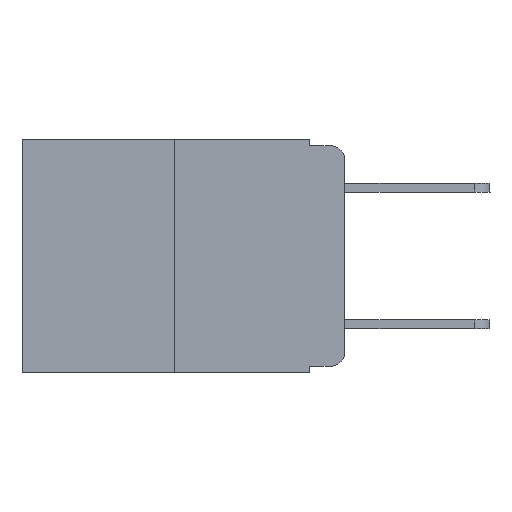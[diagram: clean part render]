
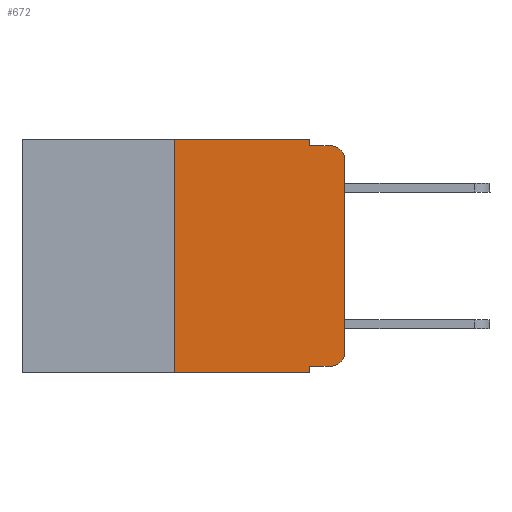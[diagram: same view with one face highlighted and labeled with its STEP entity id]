
A CAD part, left-side view. The second image highlights one B-rep face of the part: STEP entity #672.
In plain terms, the highlighted planar face has unit normal (-1, 0, 0).
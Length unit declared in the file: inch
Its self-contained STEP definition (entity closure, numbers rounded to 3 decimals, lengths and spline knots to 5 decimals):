
#62 = DIRECTION ( 'NONE',  ( 0., 0., -1. ) ) ;
#180 = DIRECTION ( 'NONE',  ( 0., -1., 0. ) ) ;
#603 = CARTESIAN_POINT ( 'NONE',  ( 0., 0.25, 0. ) ) ;
#672 = ADVANCED_FACE ( 'NONE', ( #15257 ), #4066, .F. ) ;
#681 = ORIENTED_EDGE ( 'NONE', *, *, #3427, .F. ) ;
#793 = DIRECTION ( 'NONE',  ( 0., 0., -1. ) ) ;
#1193 = DIRECTION ( 'NONE',  ( -1., 0., 0. ) ) ;
#1286 = VECTOR ( 'NONE', #15702, 39.37008 ) ;
#1287 = CARTESIAN_POINT ( 'NONE',  ( 0., 0., 0. ) ) ;
#1484 = LINE ( 'NONE', #16056, #1286 ) ;
#1562 = CARTESIAN_POINT ( 'NONE',  ( 0., 0.25, -0.343 ) ) ;
#1716 = VERTEX_POINT ( 'NONE', #8969 ) ;
#1784 = VECTOR ( 'NONE', #18478, 39.37008 ) ;
#2101 = ORIENTED_EDGE ( 'NONE', *, *, #10340, .T. ) ;
#2102 = LINE ( 'NONE', #6724, #8896 ) ;
#3020 = CARTESIAN_POINT ( 'NONE',  ( 0., 0.051, 0. ) ) ;
#3427 = EDGE_CURVE ( 'NONE', #9425, #6986, #13265, .T. ) ;
#3768 = CIRCLE ( 'NONE', #14572, 0.02 ) ;
#4066 = PLANE ( 'NONE',  #12534 ) ;
#4301 = DIRECTION ( 'NONE',  ( 0., 0., -1. ) ) ;
#4521 = DIRECTION ( 'NONE',  ( 0., 0., -1. ) ) ;
#4701 = ORIENTED_EDGE ( 'NONE', *, *, #14159, .F. ) ;
#5406 = EDGE_CURVE ( 'NONE', #7243, #9425, #1484, .T. ) ;
#5441 = AXIS2_PLACEMENT_3D ( 'NONE', #14622, #12945, #4301 ) ;
#5996 = VERTEX_POINT ( 'NONE', #9177 ) ;
#6724 = CARTESIAN_POINT ( 'NONE',  ( 0., 0.051, 0. ) ) ;
#6986 = VERTEX_POINT ( 'NONE', #16892 ) ;
#7062 = EDGE_CURVE ( 'NONE', #7435, #14889, #14156, .T. ) ;
#7243 = VERTEX_POINT ( 'NONE', #603 ) ;
#7412 = CARTESIAN_POINT ( 'NONE',  ( 0., 0.02, -0.01 ) ) ;
#7435 = VERTEX_POINT ( 'NONE', #9754 ) ;
#7472 = LINE ( 'NONE', #14248, #10600 ) ;
#7622 = LINE ( 'NONE', #11838, #1784 ) ;
#7939 = CARTESIAN_POINT ( 'NONE',  ( 0., 0., -0.03 ) ) ;
#8107 = EDGE_CURVE ( 'NONE', #14889, #14219, #15342, .T. ) ;
#8110 = DIRECTION ( 'NONE',  ( 1., 0., 0. ) ) ;
#8122 = VERTEX_POINT ( 'NONE', #1562 ) ;
#8605 = VECTOR ( 'NONE', #15674, 39.37008 ) ;
#8896 = VECTOR ( 'NONE', #793, 39.37008 ) ;
#8969 = CARTESIAN_POINT ( 'NONE',  ( 0., 0.051, -0.333 ) ) ;
#9177 = CARTESIAN_POINT ( 'NONE',  ( 0., 0.051, -0.343 ) ) ;
#9425 = VERTEX_POINT ( 'NONE', #13132 ) ;
#9754 = CARTESIAN_POINT ( 'NONE',  ( 0., 0., -0.313 ) ) ;
#9909 = EDGE_CURVE ( 'NONE', #8122, #7243, #7472, .T. ) ;
#10340 = EDGE_CURVE ( 'NONE', #8122, #5996, #7622, .T. ) ;
#10359 = ORIENTED_EDGE ( 'NONE', *, *, #14154, .T. ) ;
#10519 = CARTESIAN_POINT ( 'NONE',  ( 0., 0.051, -0.333 ) ) ;
#10600 = VECTOR ( 'NONE', #17154, 39.37008 ) ;
#11539 = CARTESIAN_POINT ( 'NONE',  ( 0., 0.02, -0.313 ) ) ;
#11838 = CARTESIAN_POINT ( 'NONE',  ( 0., 0.473, -0.343 ) ) ;
#12219 = VERTEX_POINT ( 'NONE', #15899 ) ;
#12326 = ORIENTED_EDGE ( 'NONE', *, *, #9909, .F. ) ;
#12534 = AXIS2_PLACEMENT_3D ( 'NONE', #15345, #8110, #17039 ) ;
#12676 = DIRECTION ( 'NONE',  ( 0., -1., 0. ) ) ;
#12881 = ORIENTED_EDGE ( 'NONE', *, *, #5406, .F. ) ;
#12945 = DIRECTION ( 'NONE',  ( -1., 0., 0. ) ) ;
#13132 = CARTESIAN_POINT ( 'NONE',  ( 0., 0.051, 0. ) ) ;
#13265 = LINE ( 'NONE', #3020, #14850 ) ;
#13350 = VECTOR ( 'NONE', #180, 39.37008 ) ;
#13555 = ORIENTED_EDGE ( 'NONE', *, *, #13790, .T. ) ;
#13719 = ORIENTED_EDGE ( 'NONE', *, *, #7062, .T. ) ;
#13790 = EDGE_CURVE ( 'NONE', #1716, #12219, #14834, .T. ) ;
#13984 = CARTESIAN_POINT ( 'NONE',  ( 0., 0.051, -0.01 ) ) ;
#14154 = EDGE_CURVE ( 'NONE', #12219, #7435, #3768, .T. ) ;
#14156 = LINE ( 'NONE', #1287, #8605 ) ;
#14159 = EDGE_CURVE ( 'NONE', #6986, #14219, #17264, .T. ) ;
#14219 = VERTEX_POINT ( 'NONE', #7412 ) ;
#14248 = CARTESIAN_POINT ( 'NONE',  ( 0., 0.25, 0. ) ) ;
#14362 = ORIENTED_EDGE ( 'NONE', *, *, #8107, .T. ) ;
#14572 = AXIS2_PLACEMENT_3D ( 'NONE', #11539, #1193, #62 ) ;
#14622 = CARTESIAN_POINT ( 'NONE',  ( 0., 0.02, -0.03 ) ) ;
#14834 = LINE ( 'NONE', #10519, #13350 ) ;
#14850 = VECTOR ( 'NONE', #4521, 39.37008 ) ;
#14889 = VERTEX_POINT ( 'NONE', #7939 ) ;
#15060 = ORIENTED_EDGE ( 'NONE', *, *, #16181, .F. ) ;
#15257 = FACE_OUTER_BOUND ( 'NONE', #18001, .T. ) ;
#15342 = CIRCLE ( 'NONE', #5441, 0.02 ) ;
#15345 = CARTESIAN_POINT ( 'NONE',  ( 0., 0.473, 0. ) ) ;
#15674 = DIRECTION ( 'NONE',  ( 0., 0., 1. ) ) ;
#15702 = DIRECTION ( 'NONE',  ( 0., -1., 0. ) ) ;
#15899 = CARTESIAN_POINT ( 'NONE',  ( 0., 0.02, -0.333 ) ) ;
#16056 = CARTESIAN_POINT ( 'NONE',  ( 0., 0.473, 0. ) ) ;
#16181 = EDGE_CURVE ( 'NONE', #1716, #5996, #2102, .T. ) ;
#16892 = CARTESIAN_POINT ( 'NONE',  ( 0., 0.051, -0.01 ) ) ;
#17039 = DIRECTION ( 'NONE',  ( 0., 0., -1. ) ) ;
#17154 = DIRECTION ( 'NONE',  ( 0., 0., 1. ) ) ;
#17264 = LINE ( 'NONE', #13984, #17276 ) ;
#17276 = VECTOR ( 'NONE', #12676, 39.37008 ) ;
#18001 = EDGE_LOOP ( 'NONE', ( #13719, #14362, #4701, #681, #12881, #12326, #2101, #15060, #13555, #10359 ) ) ;
#18478 = DIRECTION ( 'NONE',  ( 0., -1., 0. ) ) ;
